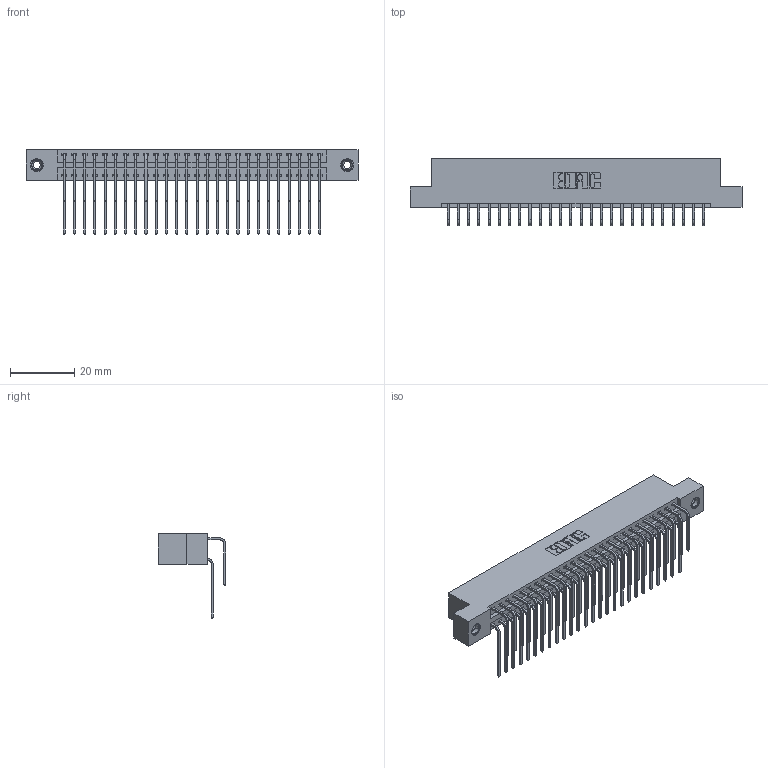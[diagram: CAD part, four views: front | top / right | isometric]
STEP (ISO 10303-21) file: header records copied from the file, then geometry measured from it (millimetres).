
FILE_DESCRIPTION (( 'STEP AP203' ), '1' );
FILE_NAME ('396-052-559-208.STEP', '2018-09-08T07:04:23', ( '' ), ( '' ), 'SwSTEP 2.0', 'SolidWorks 2016', '' );
FILE_SCHEMA (( 'CONFIG_CONTROL_DESIGN' ));
Length unit declared in the file: inch
Products named in the file (5): 346 Part_Flush Mounting Lugs - 0.156 Dia-TI; 345-292-001_558 559 Tail - 1; 345-292-001_559 Tail - 2; 345-250-001_345-250-003-102; 396-052-559-208
Assembly tree (55 placements, depth 2):
  396-052-559-208
    346 Part_Flush Mounting Lugs - 0.156 Dia-TI
    345-292-001_558 559 Tail - 1  x26
    345-292-001_559 Tail - 2  x26
    345-250-001_345-250-003-102  x2
Bounding box: 103.12 x 20.89 x 26.16 mm (x, y, z)
Volume: 10225.1 mm3; surface area: 15262.7 mm2
Topology: 55 solids, 55 shells, 2990 faces, 8837 edges, 5814 vertices
Faces by surface type: plane 2032, cylinder 942, cone 12, torus 4
Entity records: 22092 total; most frequent: CARTESIAN_POINT 3698, ORIENTED_EDGE 3574, DIRECTION 3309, EDGE_CURVE 1787, LINE 1491, VECTOR 1491, VERTEX_POINT 1184, AXIS2_PLACEMENT_3D 909
